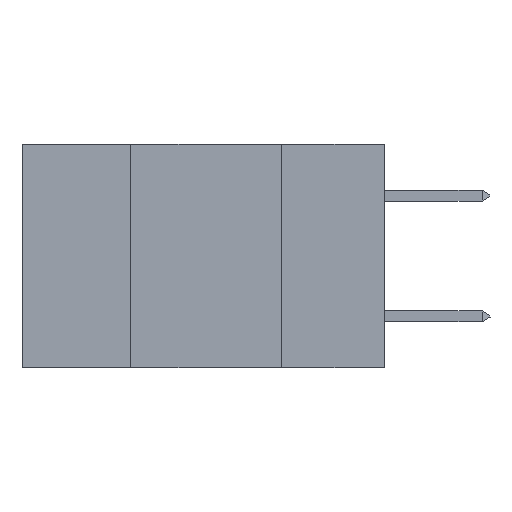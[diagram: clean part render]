
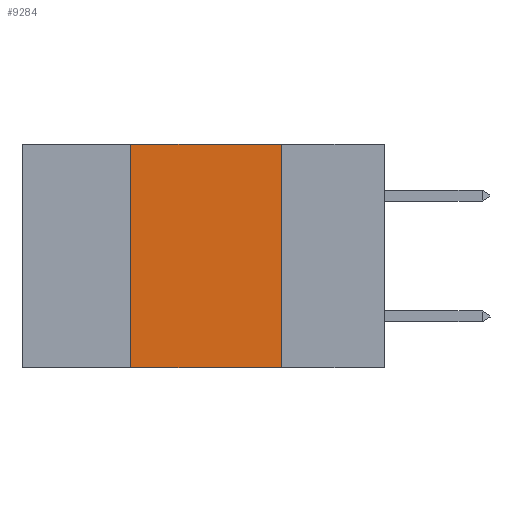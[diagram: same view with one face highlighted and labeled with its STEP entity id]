
A CAD part, left-side view. The second image highlights one B-rep face of the part: STEP entity #9284.
In plain terms, the highlighted planar face has unit normal (-1, 0, 0).
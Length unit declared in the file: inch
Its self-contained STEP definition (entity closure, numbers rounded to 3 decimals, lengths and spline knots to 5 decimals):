
#87 = CARTESIAN_POINT ( 'NONE',  ( 0., 0.6, 0. ) ) ;
#1381 = DIRECTION ( 'NONE',  ( 0., 0., 1. ) ) ;
#1864 = VECTOR ( 'NONE', #4446, 39.37008 ) ;
#2079 = VECTOR ( 'NONE', #5550, 39.37008 ) ;
#2533 = CARTESIAN_POINT ( 'NONE',  ( 0., 0.6, 0. ) ) ;
#2549 = EDGE_CURVE ( 'NONE', #13203, #3866, #8382, .T. ) ;
#3454 = CARTESIAN_POINT ( 'NONE',  ( 0., 0.17, 0. ) ) ;
#3866 = VERTEX_POINT ( 'NONE', #14715 ) ;
#4446 = DIRECTION ( 'NONE',  ( 0., -1., 0. ) ) ;
#4920 = ORIENTED_EDGE ( 'NONE', *, *, #2549, .F. ) ;
#5550 = DIRECTION ( 'NONE',  ( 0., 0., -1. ) ) ;
#5790 = EDGE_LOOP ( 'NONE', ( #7964, #6395, #4920, #11335 ) ) ;
#6035 = VERTEX_POINT ( 'NONE', #3454 ) ;
#6243 = VECTOR ( 'NONE', #1381, 39.37008 ) ;
#6395 = ORIENTED_EDGE ( 'NONE', *, *, #9507, .F. ) ;
#6822 = CARTESIAN_POINT ( 'NONE',  ( 0., 0.6, -0.37 ) ) ;
#6884 = DIRECTION ( 'NONE',  ( 0., -1., 0. ) ) ;
#7586 = CARTESIAN_POINT ( 'NONE',  ( 0., 0.42, -0.37 ) ) ;
#7964 = ORIENTED_EDGE ( 'NONE', *, *, #8831, .F. ) ;
#8382 = LINE ( 'NONE', #9556, #6243 ) ;
#8831 = EDGE_CURVE ( 'NONE', #6035, #13691, #12110, .T. ) ;
#9284 = ADVANCED_FACE ( 'NONE', ( #16977 ), #16047, .F. ) ;
#9507 = EDGE_CURVE ( 'NONE', #3866, #6035, #11059, .T. ) ;
#9556 = CARTESIAN_POINT ( 'NONE',  ( 0., 0.42, 0. ) ) ;
#9834 = CARTESIAN_POINT ( 'NONE',  ( 0., 0.17, -0.37 ) ) ;
#10567 = DIRECTION ( 'NONE',  ( 0., 0., -1. ) ) ;
#11029 = EDGE_CURVE ( 'NONE', #13203, #13691, #13284, .T. ) ;
#11059 = LINE ( 'NONE', #87, #1864 ) ;
#11335 = ORIENTED_EDGE ( 'NONE', *, *, #11029, .T. ) ;
#11403 = VECTOR ( 'NONE', #6884, 39.37008 ) ;
#12110 = LINE ( 'NONE', #13699, #2079 ) ;
#13203 = VERTEX_POINT ( 'NONE', #7586 ) ;
#13284 = LINE ( 'NONE', #6822, #11403 ) ;
#13691 = VERTEX_POINT ( 'NONE', #9834 ) ;
#13699 = CARTESIAN_POINT ( 'NONE',  ( 0., 0.17, 0. ) ) ;
#14715 = CARTESIAN_POINT ( 'NONE',  ( 0., 0.42, 0. ) ) ;
#15658 = AXIS2_PLACEMENT_3D ( 'NONE', #2533, #16236, #10567 ) ;
#16047 = PLANE ( 'NONE',  #15658 ) ;
#16236 = DIRECTION ( 'NONE',  ( 1., 0., 0. ) ) ;
#16977 = FACE_OUTER_BOUND ( 'NONE', #5790, .T. ) ;
